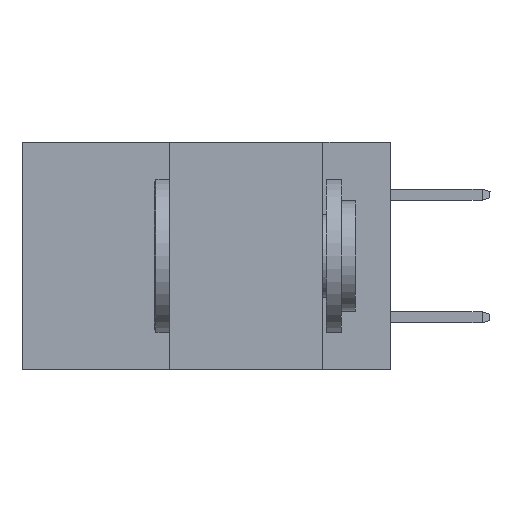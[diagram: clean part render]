
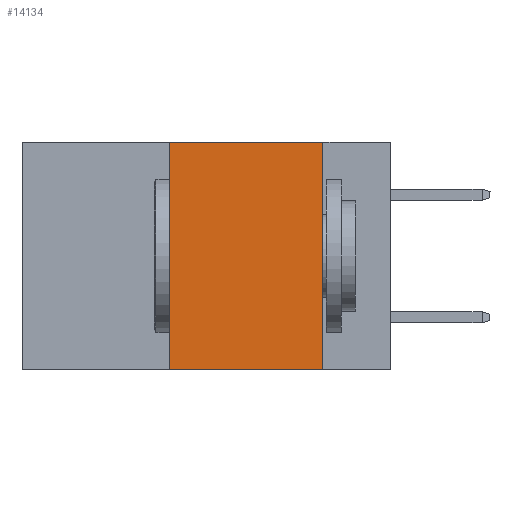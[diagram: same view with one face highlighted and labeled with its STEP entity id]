
A CAD part, left-side view. The second image highlights one B-rep face of the part: STEP entity #14134.
In plain terms, the highlighted planar face has unit normal (-1, 0, 0).
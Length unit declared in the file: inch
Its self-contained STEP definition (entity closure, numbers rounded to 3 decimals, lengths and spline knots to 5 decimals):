
#1409 = VERTEX_POINT ( 'NONE', #3448 ) ;
#1768 = CARTESIAN_POINT ( 'NONE',  ( 0., 0.36, -0.37 ) ) ;
#2392 = VERTEX_POINT ( 'NONE', #2529 ) ;
#2529 = CARTESIAN_POINT ( 'NONE',  ( 0., 0.11, 0. ) ) ;
#3374 = DIRECTION ( 'NONE',  ( 0., -1., 0. ) ) ;
#3448 = CARTESIAN_POINT ( 'NONE',  ( 0., 0.36, 0. ) ) ;
#3734 = EDGE_CURVE ( 'NONE', #7780, #1409, #14298, .T. ) ;
#3867 = AXIS2_PLACEMENT_3D ( 'NONE', #9694, #11229, #14392 ) ;
#3923 = CARTESIAN_POINT ( 'NONE',  ( 0., 0.36, 0. ) ) ;
#4524 = DIRECTION ( 'NONE',  ( 0., 0., -1. ) ) ;
#5282 = ORIENTED_EDGE ( 'NONE', *, *, #3734, .F. ) ;
#5504 = VECTOR ( 'NONE', #7562, 39.37008 ) ;
#6021 = VERTEX_POINT ( 'NONE', #11412 ) ;
#6326 = ORIENTED_EDGE ( 'NONE', *, *, #14182, .F. ) ;
#7562 = DIRECTION ( 'NONE',  ( 0., 0., 1. ) ) ;
#7669 = DIRECTION ( 'NONE',  ( 0., -1., 0. ) ) ;
#7780 = VERTEX_POINT ( 'NONE', #1768 ) ;
#9694 = CARTESIAN_POINT ( 'NONE',  ( 0., 0.6, 0. ) ) ;
#10313 = LINE ( 'NONE', #13385, #10826 ) ;
#10826 = VECTOR ( 'NONE', #3374, 39.37008 ) ;
#11229 = DIRECTION ( 'NONE',  ( 1., 0., 0. ) ) ;
#11412 = CARTESIAN_POINT ( 'NONE',  ( 0., 0.11, -0.37 ) ) ;
#11434 = FACE_OUTER_BOUND ( 'NONE', #15768, .T. ) ;
#12177 = VECTOR ( 'NONE', #7669, 39.37008 ) ;
#12460 = EDGE_CURVE ( 'NONE', #7780, #6021, #10313, .T. ) ;
#12702 = VECTOR ( 'NONE', #4524, 39.37008 ) ;
#13039 = LINE ( 'NONE', #14321, #12177 ) ;
#13385 = CARTESIAN_POINT ( 'NONE',  ( 0., 0.6, -0.37 ) ) ;
#14134 = ADVANCED_FACE ( 'NONE', ( #11434 ), #19557, .F. ) ;
#14182 = EDGE_CURVE ( 'NONE', #2392, #6021, #19736, .T. ) ;
#14298 = LINE ( 'NONE', #3923, #5504 ) ;
#14321 = CARTESIAN_POINT ( 'NONE',  ( 0., 0.6, 0. ) ) ;
#14392 = DIRECTION ( 'NONE',  ( 0., 0., -1. ) ) ;
#14473 = CARTESIAN_POINT ( 'NONE',  ( 0., 0.11, 0. ) ) ;
#15768 = EDGE_LOOP ( 'NONE', ( #6326, #16113, #5282, #17557 ) ) ;
#16113 = ORIENTED_EDGE ( 'NONE', *, *, #20848, .F. ) ;
#17557 = ORIENTED_EDGE ( 'NONE', *, *, #12460, .T. ) ;
#19557 = PLANE ( 'NONE',  #3867 ) ;
#19736 = LINE ( 'NONE', #14473, #12702 ) ;
#20848 = EDGE_CURVE ( 'NONE', #1409, #2392, #13039, .T. ) ;
